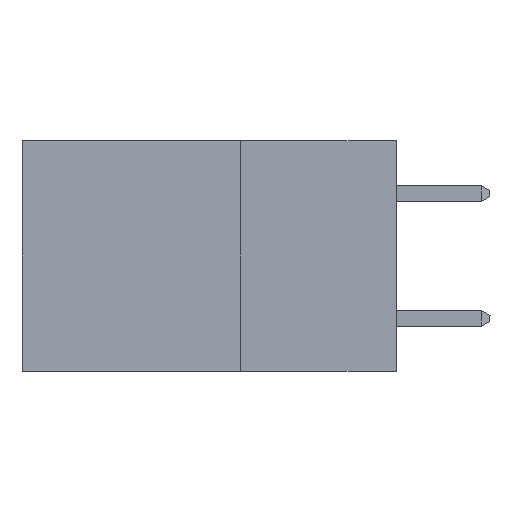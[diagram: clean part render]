
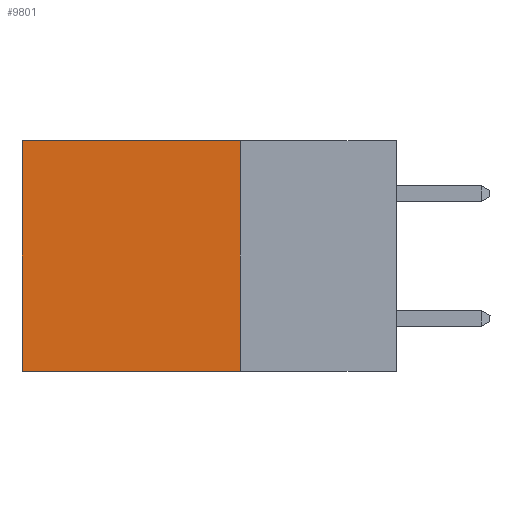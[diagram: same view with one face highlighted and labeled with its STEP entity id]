
A CAD part, left-side view. The second image highlights one B-rep face of the part: STEP entity #9801.
In plain terms, the highlighted planar face has unit normal (-1, 0, 0).
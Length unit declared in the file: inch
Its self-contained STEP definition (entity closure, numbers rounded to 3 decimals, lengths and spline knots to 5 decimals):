
#118 = ORIENTED_EDGE ( 'NONE', *, *, #4339, .F. ) ;
#785 = VERTEX_POINT ( 'NONE', #10560 ) ;
#915 = EDGE_CURVE ( 'NONE', #3102, #6226, #11694, .T. ) ;
#987 = DIRECTION ( 'NONE',  ( 0., 1., 0. ) ) ;
#1094 = VERTEX_POINT ( 'NONE', #7831 ) ;
#1279 = DIRECTION ( 'NONE',  ( 0., 0., -1. ) ) ;
#1803 = CARTESIAN_POINT ( 'NONE',  ( 0.298, 0.25, 0. ) ) ;
#1858 = LINE ( 'NONE', #4625, #4290 ) ;
#2158 = EDGE_CURVE ( 'NONE', #3102, #785, #1858, .T. ) ;
#3027 = VECTOR ( 'NONE', #1279, 39.37008 ) ;
#3102 = VERTEX_POINT ( 'NONE', #1803 ) ;
#3682 = CARTESIAN_POINT ( 'NONE',  ( 0.298, 0.25, -0.37 ) ) ;
#3730 = CARTESIAN_POINT ( 'NONE',  ( 0.298, 0.25, -0.37 ) ) ;
#4290 = VECTOR ( 'NONE', #987, 39.37008 ) ;
#4339 = EDGE_CURVE ( 'NONE', #6226, #1094, #6912, .T. ) ;
#4386 = ORIENTED_EDGE ( 'NONE', *, *, #915, .F. ) ;
#4432 = DIRECTION ( 'NONE',  ( 1., 0., 0. ) ) ;
#4486 = VECTOR ( 'NONE', #11095, 39.37008 ) ;
#4492 = CARTESIAN_POINT ( 'NONE',  ( 0.298, 0.6, 0. ) ) ;
#4625 = CARTESIAN_POINT ( 'NONE',  ( 0.298, 0.25, 0. ) ) ;
#5573 = VECTOR ( 'NONE', #11750, 39.37008 ) ;
#5660 = AXIS2_PLACEMENT_3D ( 'NONE', #9859, #4432, #7147 ) ;
#6164 = LINE ( 'NONE', #4492, #5573 ) ;
#6173 = EDGE_CURVE ( 'NONE', #785, #1094, #6164, .T. ) ;
#6226 = VERTEX_POINT ( 'NONE', #3682 ) ;
#6912 = LINE ( 'NONE', #3730, #4486 ) ;
#7147 = DIRECTION ( 'NONE',  ( 0., 0., -1. ) ) ;
#7346 = EDGE_LOOP ( 'NONE', ( #10429, #118, #4386, #11589 ) ) ;
#7831 = CARTESIAN_POINT ( 'NONE',  ( 0.298, 0.6, -0.37 ) ) ;
#8485 = CARTESIAN_POINT ( 'NONE',  ( 0.298, 0.25, 0. ) ) ;
#9801 = ADVANCED_FACE ( 'NONE', ( #11125 ), #11652, .F. ) ;
#9859 = CARTESIAN_POINT ( 'NONE',  ( 0.298, 0.25, 0. ) ) ;
#10429 = ORIENTED_EDGE ( 'NONE', *, *, #6173, .T. ) ;
#10560 = CARTESIAN_POINT ( 'NONE',  ( 0.298, 0.6, 0. ) ) ;
#11095 = DIRECTION ( 'NONE',  ( 0., 1., 0. ) ) ;
#11125 = FACE_OUTER_BOUND ( 'NONE', #7346, .T. ) ;
#11589 = ORIENTED_EDGE ( 'NONE', *, *, #2158, .T. ) ;
#11652 = PLANE ( 'NONE',  #5660 ) ;
#11694 = LINE ( 'NONE', #8485, #3027 ) ;
#11750 = DIRECTION ( 'NONE',  ( 0., 0., -1. ) ) ;
